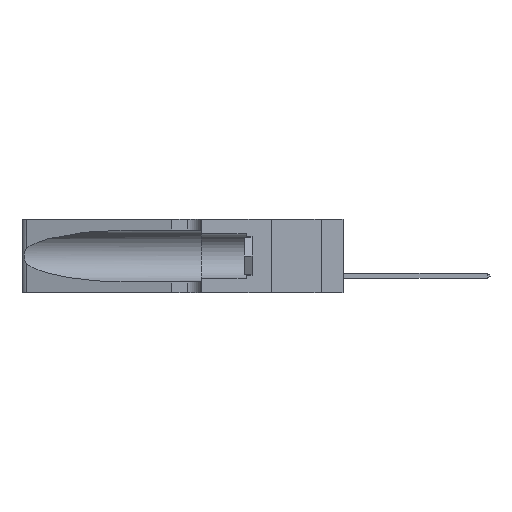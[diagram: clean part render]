
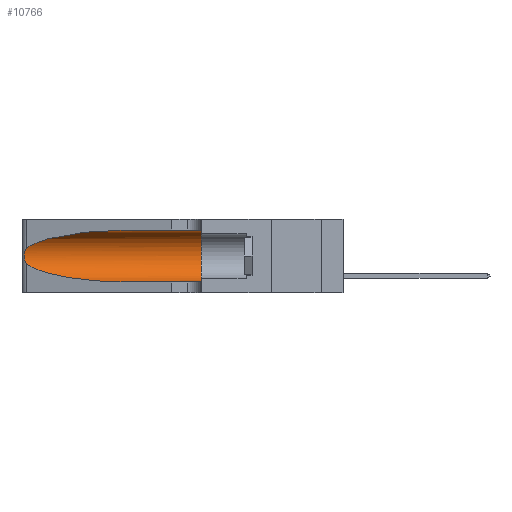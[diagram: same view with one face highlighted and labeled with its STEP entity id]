
A CAD part, left-side view. The second image highlights one B-rep face of the part: STEP entity #10766.
In plain terms, the highlighted cylindrical face has radius 3.308 mm (diameter 6.617 mm), a partial arc.
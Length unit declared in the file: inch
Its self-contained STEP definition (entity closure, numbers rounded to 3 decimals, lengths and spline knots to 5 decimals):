
#291 = ORIENTED_EDGE ( 'NONE', *, *, #17153, .T. ) ;
#370 = EDGE_LOOP ( 'NONE', ( #5174, #291, #10725, #20950, #9285, #20824 ) ) ;
#475 = CARTESIAN_POINT ( 'NONE',  ( 0.25787, 1.23484, 0.2124 ) ) ;
#1232 = VECTOR ( 'NONE', #20422, 39.37008 ) ;
#1559 = DIRECTION ( 'NONE',  ( 0., -1., 0. ) ) ;
#1870 = CARTESIAN_POINT ( 'NONE',  ( 0.25639, 1.23186, 0.15144 ) ) ;
#1940 = CARTESIAN_POINT ( 'NONE',  ( 0.25856, 1.23593, 0.16098 ) ) ;
#1964 = VERTEX_POINT ( 'NONE', #11289 ) ;
#2093 = FACE_OUTER_BOUND ( 'NONE', #370, .T. ) ;
#2104 = EDGE_CURVE ( 'NONE', #17547, #15935, #16737, .T. ) ;
#2544 = CARTESIAN_POINT ( 'NONE',  ( 0.1305, 1.61858, 0.185 ) ) ;
#3052 = AXIS2_PLACEMENT_3D ( 'NONE', #4524, #16529, #5309 ) ;
#3647 = CARTESIAN_POINT ( 'NONE',  ( 0.25789, 1.23486, 0.15765 ) ) ;
#3938 =( BOUNDED_CURVE ( )  B_SPLINE_CURVE ( 3, ( #16752, #8306, #22028, #15316 ),
 .UNSPECIFIED., .F., .T. ) 
 B_SPLINE_CURVE_WITH_KNOTS ( ( 4, 4 ),
 ( 1.5708, 2.84003 ),
 .UNSPECIFIED. ) 
 CURVE ( )  GEOMETRIC_REPRESENTATION_ITEM ( )  RATIONAL_B_SPLINE_CURVE ( ( 1., 0.87, 0.87, 1. ) ) 
 REPRESENTATION_ITEM ( '' )  );
#4524 = CARTESIAN_POINT ( 'NONE',  ( 0.1305, 0.35, 0.185 ) ) ;
#4583 = CARTESIAN_POINT ( 'NONE',  ( 0.25555, 1.22994, 0.2215 ) ) ;
#5174 = ORIENTED_EDGE ( 'NONE', *, *, #9922, .T. ) ;
#5309 = DIRECTION ( 'NONE',  ( 0., 0., 1. ) ) ;
#5516 = CARTESIAN_POINT ( 'NONE',  ( 0.25854, 1.2359, 0.20912 ) ) ;
#5816 = DIRECTION ( 'NONE',  ( 0., -1., 0. ) ) ;
#6170 = CARTESIAN_POINT ( 'NONE',  ( 0.25487, 1.22718, 0.22369 ) ) ;
#7719 = DIRECTION ( 'NONE',  ( 0., 0., -1. ) ) ;
#8110 = CARTESIAN_POINT ( 'NONE',  ( 0.2373, 1.15595, 0.08982 ) ) ;
#8306 = CARTESIAN_POINT ( 'NONE',  ( 0.18966, 0.96281, 0.31525 ) ) ;
#8398 = CARTESIAN_POINT ( 'NONE',  ( 0.1305, 0.35, 0.31525 ) ) ;
#8687 = CARTESIAN_POINT ( 'NONE',  ( 0.26018, 1.23835, 0.19895 ) ) ;
#8740 = LINE ( 'NONE', #11894, #1232 ) ;
#8853 = CARTESIAN_POINT ( 'NONE',  ( 0.26075, 1.23896, 0.19203 ) ) ;
#9285 = ORIENTED_EDGE ( 'NONE', *, *, #17955, .F. ) ;
#9457 = EDGE_CURVE ( 'NONE', #16590, #22138, #11638, .T. ) ;
#9649 = CARTESIAN_POINT ( 'NONE',  ( 0.25639, 1.23184, 0.21858 ) ) ;
#9862 = CARTESIAN_POINT ( 'NONE',  ( 0.1305, 0.72297, 0.05475 ) ) ;
#9922 = EDGE_CURVE ( 'NONE', #17547, #1964, #3938, .T. ) ;
#10725 = ORIENTED_EDGE ( 'NONE', *, *, #9457, .T. ) ;
#10766 = ADVANCED_FACE ( 'NONE', ( #2093 ), #12284, .F. ) ;
#11289 = CARTESIAN_POINT ( 'NONE',  ( 0.25487, 1.22718, 0.22369 ) ) ;
#11339 = VERTEX_POINT ( 'NONE', #18174 ) ;
#11554 = CARTESIAN_POINT ( 'NONE',  ( 0.25487, 1.22718, 0.14631 ) ) ;
#11638 =( BOUNDED_CURVE ( )  B_SPLINE_CURVE ( 3, ( #11554, #8110, #18413, #9862 ),
 .UNSPECIFIED., .F., .T. ) 
 B_SPLINE_CURVE_WITH_KNOTS ( ( 4, 4 ),
 ( 3.44316, 4.71239 ),
 .UNSPECIFIED. ) 
 CURVE ( )  GEOMETRIC_REPRESENTATION_ITEM ( )  RATIONAL_B_SPLINE_CURVE ( ( 1., 0.87, 0.87, 1. ) ) 
 REPRESENTATION_ITEM ( '' )  );
#11704 = CARTESIAN_POINT ( 'NONE',  ( 0.1305, 0.72297, 0.05475 ) ) ;
#11822 = CARTESIAN_POINT ( 'NONE',  ( 0.1305, 1.61858, 0.31525 ) ) ;
#11894 = CARTESIAN_POINT ( 'NONE',  ( 0.1305, 1.61858, 0.05475 ) ) ;
#12223 = VECTOR ( 'NONE', #1559, 39.37008 ) ;
#12284 = CYLINDRICAL_SURFACE ( 'NONE', #19022, 0.13025 ) ;
#13144 = CARTESIAN_POINT ( 'NONE',  ( 0.25487, 1.22718, 0.14631 ) ) ;
#13917 = CARTESIAN_POINT ( 'NONE',  ( 0.26017, 1.23833, 0.17102 ) ) ;
#15101 = CARTESIAN_POINT ( 'NONE',  ( 0.1305, 0.72297, 0.31525 ) ) ;
#15316 = CARTESIAN_POINT ( 'NONE',  ( 0.25487, 1.22718, 0.22369 ) ) ;
#15629 = CARTESIAN_POINT ( 'NONE',  ( 0.25487, 1.22718, 0.14631 ) ) ;
#15786 = CARTESIAN_POINT ( 'NONE',  ( 0.26075, 1.23896, 0.178 ) ) ;
#15935 = VERTEX_POINT ( 'NONE', #8398 ) ;
#16529 = DIRECTION ( 'NONE',  ( 0., 1., 0. ) ) ;
#16590 = VERTEX_POINT ( 'NONE', #13144 ) ;
#16737 = LINE ( 'NONE', #11822, #12223 ) ;
#16752 = CARTESIAN_POINT ( 'NONE',  ( 0.1305, 0.72297, 0.31525 ) ) ;
#17153 = EDGE_CURVE ( 'NONE', #1964, #16590, #18226, .T. ) ;
#17547 = VERTEX_POINT ( 'NONE', #15101 ) ;
#17955 = EDGE_CURVE ( 'NONE', #15935, #11339, #18206, .T. ) ;
#18174 = CARTESIAN_POINT ( 'NONE',  ( 0.1305, 0.35, 0.05475 ) ) ;
#18206 = CIRCLE ( 'NONE', #3052, 0.13025 ) ;
#18226 = B_SPLINE_CURVE_WITH_KNOTS ( 'NONE', 3,
 ( #6170, #4583, #9649, #475, #5516, #8687, #8853, #15786, #13917, #1940, #3647, #1870, #20650, #15629 ),
 .UNSPECIFIED., .F., .F.,
 ( 4, 2, 2, 2, 2, 2, 4 ),
 ( 0., 0.00027, 0.00053, 0.00107, 0.0016, 0.00187, 0.00214 ),
 .UNSPECIFIED. ) ;
#18413 = CARTESIAN_POINT ( 'NONE',  ( 0.18966, 0.96281, 0.05475 ) ) ;
#19022 = AXIS2_PLACEMENT_3D ( 'NONE', #2544, #5816, #7719 ) ;
#20422 = DIRECTION ( 'NONE',  ( 0., -1., 0. ) ) ;
#20650 = CARTESIAN_POINT ( 'NONE',  ( 0.25555, 1.22993, 0.14849 ) ) ;
#20780 = EDGE_CURVE ( 'NONE', #22138, #11339, #8740, .T. ) ;
#20824 = ORIENTED_EDGE ( 'NONE', *, *, #2104, .F. ) ;
#20950 = ORIENTED_EDGE ( 'NONE', *, *, #20780, .T. ) ;
#22028 = CARTESIAN_POINT ( 'NONE',  ( 0.2373, 1.15595, 0.28018 ) ) ;
#22138 = VERTEX_POINT ( 'NONE', #11704 ) ;
